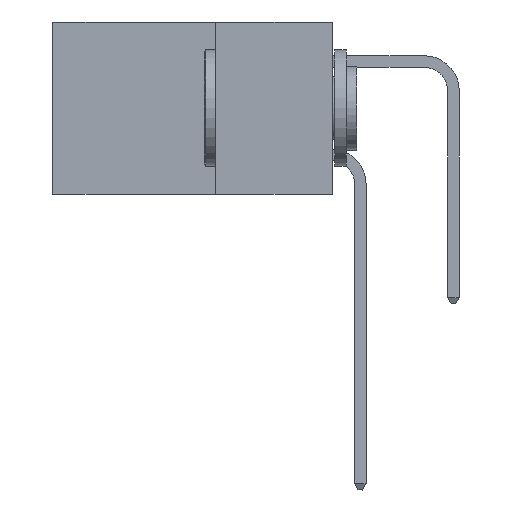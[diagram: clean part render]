
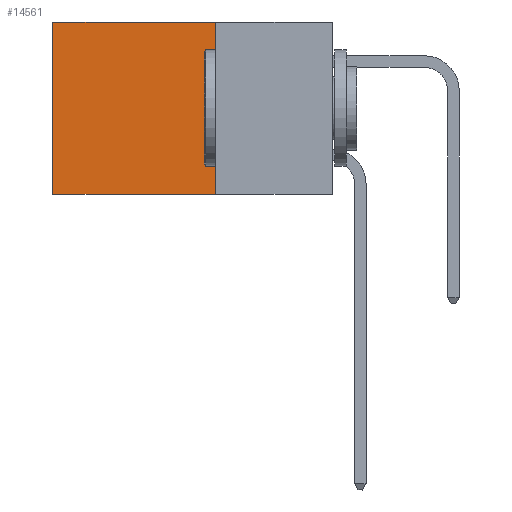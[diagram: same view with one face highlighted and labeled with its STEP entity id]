
A CAD part, left-side view. The second image highlights one B-rep face of the part: STEP entity #14561.
In plain terms, the highlighted planar face has unit normal (-1, 0, 0).
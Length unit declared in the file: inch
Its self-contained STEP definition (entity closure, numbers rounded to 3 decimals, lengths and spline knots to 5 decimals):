
#199 = ORIENTED_EDGE ( 'NONE', *, *, #4985, .T. ) ;
#703 = DIRECTION ( 'NONE',  ( 1., 0., 0. ) ) ;
#1316 = CARTESIAN_POINT ( 'NONE',  ( 0.2615, 0.6, 0. ) ) ;
#1446 = VERTEX_POINT ( 'NONE', #4031 ) ;
#1550 = VECTOR ( 'NONE', #6030, 39.37008 ) ;
#1711 = ORIENTED_EDGE ( 'NONE', *, *, #14080, .F. ) ;
#2314 = PLANE ( 'NONE',  #2377 ) ;
#2377 = AXIS2_PLACEMENT_3D ( 'NONE', #11401, #703, #8404 ) ;
#3132 = EDGE_CURVE ( 'NONE', #1446, #10839, #13200, .T. ) ;
#4031 = CARTESIAN_POINT ( 'NONE',  ( 0.2615, 0.25, 0. ) ) ;
#4629 = ORIENTED_EDGE ( 'NONE', *, *, #3132, .F. ) ;
#4985 = EDGE_CURVE ( 'NONE', #17419, #18520, #17301, .T. ) ;
#5053 = LINE ( 'NONE', #15819, #17389 ) ;
#6030 = DIRECTION ( 'NONE',  ( 0., 1., 0. ) ) ;
#7401 = CARTESIAN_POINT ( 'NONE',  ( 0.2615, 0.25, -0.37 ) ) ;
#8242 = CARTESIAN_POINT ( 'NONE',  ( 0.2615, 0.6, -0.37 ) ) ;
#8334 = DIRECTION ( 'NONE',  ( 0., 0., -1. ) ) ;
#8404 = DIRECTION ( 'NONE',  ( 0., 0., -1. ) ) ;
#9014 = CARTESIAN_POINT ( 'NONE',  ( 0.2615, 0.25, 0. ) ) ;
#9109 = ORIENTED_EDGE ( 'NONE', *, *, #9358, .T. ) ;
#9358 = EDGE_CURVE ( 'NONE', #1446, #17419, #17991, .T. ) ;
#10839 = VERTEX_POINT ( 'NONE', #11128 ) ;
#11128 = CARTESIAN_POINT ( 'NONE',  ( 0.2615, 0.25, -0.37 ) ) ;
#11401 = CARTESIAN_POINT ( 'NONE',  ( 0.2615, 0.25, -0.37 ) ) ;
#12911 = FACE_OUTER_BOUND ( 'NONE', #17580, .T. ) ;
#13200 = LINE ( 'NONE', #7401, #15800 ) ;
#13474 = DIRECTION ( 'NONE',  ( 0., 0., -1. ) ) ;
#14080 = EDGE_CURVE ( 'NONE', #10839, #18520, #5053, .T. ) ;
#14561 = ADVANCED_FACE ( 'NONE', ( #12911 ), #2314, .F. ) ;
#15800 = VECTOR ( 'NONE', #13474, 39.37008 ) ;
#15819 = CARTESIAN_POINT ( 'NONE',  ( 0.2615, 0.25, -0.37 ) ) ;
#16298 = CARTESIAN_POINT ( 'NONE',  ( 0.2615, 0.6, -0.37 ) ) ;
#16884 = VECTOR ( 'NONE', #8334, 39.37008 ) ;
#17292 = DIRECTION ( 'NONE',  ( 0., 1., 0. ) ) ;
#17301 = LINE ( 'NONE', #8242, #16884 ) ;
#17389 = VECTOR ( 'NONE', #17292, 39.37008 ) ;
#17419 = VERTEX_POINT ( 'NONE', #1316 ) ;
#17580 = EDGE_LOOP ( 'NONE', ( #199, #1711, #4629, #9109 ) ) ;
#17991 = LINE ( 'NONE', #9014, #1550 ) ;
#18520 = VERTEX_POINT ( 'NONE', #16298 ) ;
